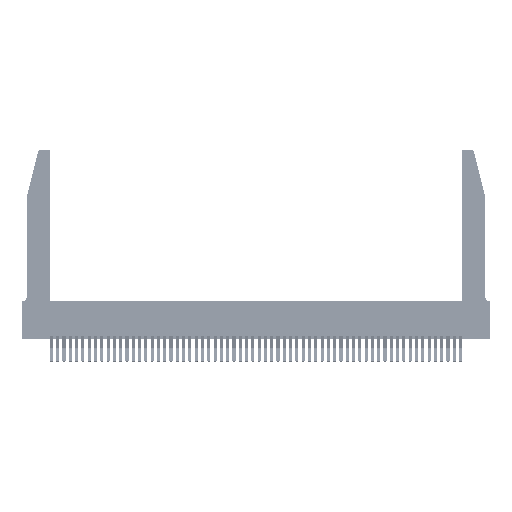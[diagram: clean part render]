
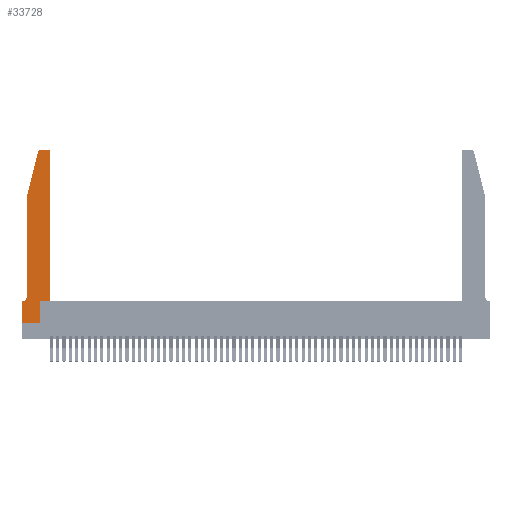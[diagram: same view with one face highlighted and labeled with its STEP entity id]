
A CAD part, top view. The second image highlights one B-rep face of the part: STEP entity #33728.
In plain terms, the highlighted planar face has unit normal (0, 0, 1).
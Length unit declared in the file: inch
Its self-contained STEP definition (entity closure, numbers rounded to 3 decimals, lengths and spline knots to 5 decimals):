
#381 = CARTESIAN_POINT ( 'NONE',  ( 0.2605, 2.75, 0.37 ) ) ;
#389 = VERTEX_POINT ( 'NONE', #47157 ) ;
#446 = EDGE_LOOP ( 'NONE', ( #33471, #7596, #6288, #51975, #35978, #28278, #13360, #5556, #51272, #18550, #3567, #45477 ) ) ;
#621 = DIRECTION ( 'NONE',  ( 1., 0., 0. ) ) ;
#2139 = VECTOR ( 'NONE', #31481, 39.37008 ) ;
#2301 = CARTESIAN_POINT ( 'NONE',  ( 0.0755, 2., 0.37 ) ) ;
#2329 = DIRECTION ( 'NONE',  ( 0., -1., 0. ) ) ;
#3567 = ORIENTED_EDGE ( 'NONE', *, *, #33886, .T. ) ;
#4329 = CIRCLE ( 'NONE', #40291, 0.07 ) ;
#4392 = EDGE_CURVE ( 'NONE', #389, #42416, #26223, .T. ) ;
#4861 = CIRCLE ( 'NONE', #6751, 0.03 ) ;
#5556 = ORIENTED_EDGE ( 'NONE', *, *, #8023, .T. ) ;
#5686 = CARTESIAN_POINT ( 'NONE',  ( 0.0755, 2., 0.37 ) ) ;
#5728 = LINE ( 'NONE', #34584, #37371 ) ;
#6198 = EDGE_CURVE ( 'NONE', #42653, #25215, #35159, .T. ) ;
#6288 = ORIENTED_EDGE ( 'NONE', *, *, #42700, .T. ) ;
#6518 = EDGE_CURVE ( 'NONE', #7917, #10982, #31959, .T. ) ;
#6751 = AXIS2_PLACEMENT_3D ( 'NONE', #12200, #41031, #16345 ) ;
#7596 = ORIENTED_EDGE ( 'NONE', *, *, #47562, .T. ) ;
#7881 = VECTOR ( 'NONE', #40955, 39.37008 ) ;
#7917 = VERTEX_POINT ( 'NONE', #31753 ) ;
#8023 = EDGE_CURVE ( 'NONE', #16915, #42832, #25317, .T. ) ;
#8408 = EDGE_CURVE ( 'NONE', #42416, #16915, #43689, .T. ) ;
#8581 = VERTEX_POINT ( 'NONE', #40481 ) ;
#8644 = VECTOR ( 'NONE', #37697, 39.37008 ) ;
#9061 = CARTESIAN_POINT ( 'NONE',  ( 0.4505, 0.35, 0.37 ) ) ;
#10982 = VERTEX_POINT ( 'NONE', #30411 ) ;
#11407 = VECTOR ( 'NONE', #17372, 39.37008 ) ;
#12200 = CARTESIAN_POINT ( 'NONE',  ( 0.4205, 2.72, 0.37 ) ) ;
#13200 = CARTESIAN_POINT ( 'NONE',  ( 0.2865, 0.35, 0.37 ) ) ;
#13360 = ORIENTED_EDGE ( 'NONE', *, *, #8408, .T. ) ;
#14456 = EDGE_CURVE ( 'NONE', #25215, #389, #4329, .T. ) ;
#14720 = CARTESIAN_POINT ( 'NONE',  ( 0., 0., 0.37 ) ) ;
#14811 = DIRECTION ( 'NONE',  ( 0., 0., 1. ) ) ;
#15497 = EDGE_CURVE ( 'NONE', #15524, #7917, #4861, .T. ) ;
#15524 = VERTEX_POINT ( 'NONE', #28817 ) ;
#16028 = CARTESIAN_POINT ( 'NONE',  ( 0., 0., 0.37 ) ) ;
#16195 = DIRECTION ( 'NONE',  ( 1., 0., 0. ) ) ;
#16345 = DIRECTION ( 'NONE',  ( 1., 0., 0. ) ) ;
#16915 = VERTEX_POINT ( 'NONE', #18260 ) ;
#17372 = DIRECTION ( 'NONE',  ( 0., 1., 0. ) ) ;
#17904 = DIRECTION ( 'NONE',  ( 0., 0., -1. ) ) ;
#18224 = DIRECTION ( 'NONE',  ( -0.239, -0.971, 0. ) ) ;
#18260 = CARTESIAN_POINT ( 'NONE',  ( 0., 0., 0.37 ) ) ;
#18550 = ORIENTED_EDGE ( 'NONE', *, *, #28085, .T. ) ;
#19413 = PLANE ( 'NONE',  #42649 ) ;
#20487 = CARTESIAN_POINT ( 'NONE',  ( 0.4505, 0.35, 0.37 ) ) ;
#22787 = VECTOR ( 'NONE', #16195, 39.37008 ) ;
#23552 = DIRECTION ( 'NONE',  ( 0., 0., 1. ) ) ;
#25215 = VERTEX_POINT ( 'NONE', #40368 ) ;
#25317 = LINE ( 'NONE', #16028, #22787 ) ;
#25318 = VERTEX_POINT ( 'NONE', #49622 ) ;
#26223 = LINE ( 'NONE', #28257, #35834 ) ;
#27012 = LINE ( 'NONE', #9061, #28308 ) ;
#27419 = CARTESIAN_POINT ( 'NONE',  ( 0.25487, 2.72718, 0.37 ) ) ;
#28085 = EDGE_CURVE ( 'NONE', #8581, #25318, #27012, .T. ) ;
#28257 = CARTESIAN_POINT ( 'NONE',  ( 0.0755, 0.35, 0.37 ) ) ;
#28278 = ORIENTED_EDGE ( 'NONE', *, *, #4392, .T. ) ;
#28308 = VECTOR ( 'NONE', #621, 39.37008 ) ;
#28817 = CARTESIAN_POINT ( 'NONE',  ( 0.4505, 2.72, 0.37 ) ) ;
#30411 = CARTESIAN_POINT ( 'NONE',  ( 0.284, 2.75, 0.37 ) ) ;
#31481 = DIRECTION ( 'NONE',  ( 0., -1., 0. ) ) ;
#31753 = CARTESIAN_POINT ( 'NONE',  ( 0.4205, 2.75, 0.37 ) ) ;
#31959 = LINE ( 'NONE', #381, #8644 ) ;
#32061 = AXIS2_PLACEMENT_3D ( 'NONE', #39494, #14811, #43623 ) ;
#33025 = CARTESIAN_POINT ( 'NONE',  ( 0., 0.35, 0.37 ) ) ;
#33361 = LINE ( 'NONE', #13200, #11407 ) ;
#33471 = ORIENTED_EDGE ( 'NONE', *, *, #6518, .T. ) ;
#33728 = ADVANCED_FACE ( 'NONE', ( #37594 ), #19413, .T. ) ;
#33820 = CIRCLE ( 'NONE', #32061, 0.03 ) ;
#33886 = EDGE_CURVE ( 'NONE', #25318, #15524, #40815, .T. ) ;
#34584 = CARTESIAN_POINT ( 'NONE',  ( 0.0755, 2., 0.37 ) ) ;
#35159 = LINE ( 'NONE', #2301, #2139 ) ;
#35834 = VECTOR ( 'NONE', #48868, 39.37008 ) ;
#35978 = ORIENTED_EDGE ( 'NONE', *, *, #14456, .T. ) ;
#36787 = VERTEX_POINT ( 'NONE', #27419 ) ;
#37371 = VECTOR ( 'NONE', #18224, 39.37008 ) ;
#37594 = FACE_OUTER_BOUND ( 'NONE', #446, .T. ) ;
#37697 = DIRECTION ( 'NONE',  ( -1., 0., 0. ) ) ;
#38443 = EDGE_CURVE ( 'NONE', #42832, #8581, #33361, .T. ) ;
#38796 = VECTOR ( 'NONE', #2329, 39.37008 ) ;
#39494 = CARTESIAN_POINT ( 'NONE',  ( 0.284, 2.72, 0.37 ) ) ;
#40291 = AXIS2_PLACEMENT_3D ( 'NONE', #42534, #17904, #46638 ) ;
#40368 = CARTESIAN_POINT ( 'NONE',  ( 0.0755, 0.42, 0.37 ) ) ;
#40481 = CARTESIAN_POINT ( 'NONE',  ( 0.2865, 0.35, 0.37 ) ) ;
#40815 = LINE ( 'NONE', #20487, #7881 ) ;
#40955 = DIRECTION ( 'NONE',  ( 0., 1., 0. ) ) ;
#41031 = DIRECTION ( 'NONE',  ( 0., 0., 1. ) ) ;
#42416 = VERTEX_POINT ( 'NONE', #33025 ) ;
#42534 = CARTESIAN_POINT ( 'NONE',  ( 0.0055, 0.42, 0.37 ) ) ;
#42649 = AXIS2_PLACEMENT_3D ( 'NONE', #44018, #23552, #52190 ) ;
#42653 = VERTEX_POINT ( 'NONE', #5686 ) ;
#42700 = EDGE_CURVE ( 'NONE', #36787, #42653, #5728, .T. ) ;
#42832 = VERTEX_POINT ( 'NONE', #47676 ) ;
#43623 = DIRECTION ( 'NONE',  ( 1., 0., 0. ) ) ;
#43689 = LINE ( 'NONE', #14720, #38796 ) ;
#44018 = CARTESIAN_POINT ( 'NONE',  ( 0., 0.35, 0.37 ) ) ;
#45477 = ORIENTED_EDGE ( 'NONE', *, *, #15497, .T. ) ;
#46638 = DIRECTION ( 'NONE',  ( -1., 0., 0. ) ) ;
#47157 = CARTESIAN_POINT ( 'NONE',  ( 0.0055, 0.35, 0.37 ) ) ;
#47562 = EDGE_CURVE ( 'NONE', #10982, #36787, #33820, .T. ) ;
#47676 = CARTESIAN_POINT ( 'NONE',  ( 0.2865, 0., 0.37 ) ) ;
#48868 = DIRECTION ( 'NONE',  ( -1., 0., 0. ) ) ;
#49622 = CARTESIAN_POINT ( 'NONE',  ( 0.4505, 0.35, 0.37 ) ) ;
#51272 = ORIENTED_EDGE ( 'NONE', *, *, #38443, .T. ) ;
#51975 = ORIENTED_EDGE ( 'NONE', *, *, #6198, .T. ) ;
#52190 = DIRECTION ( 'NONE',  ( 1., 0., 0. ) ) ;
